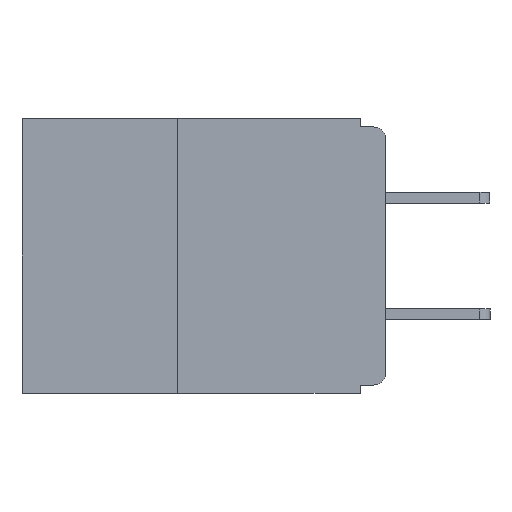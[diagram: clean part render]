
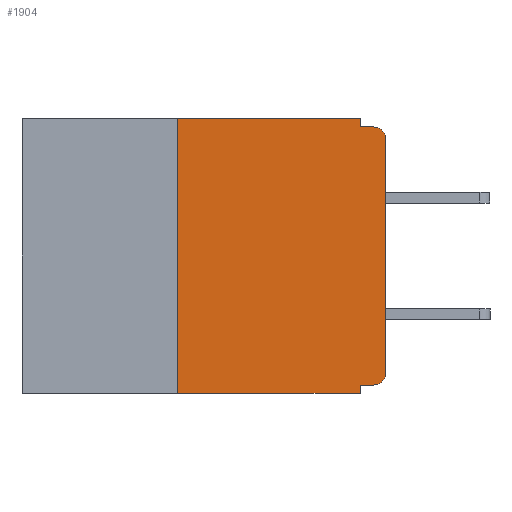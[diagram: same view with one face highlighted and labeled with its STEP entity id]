
A CAD part, left-side view. The second image highlights one B-rep face of the part: STEP entity #1904.
In plain terms, the highlighted planar face has unit normal (-1, 0, 0).
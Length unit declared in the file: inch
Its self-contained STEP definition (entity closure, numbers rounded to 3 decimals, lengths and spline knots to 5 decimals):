
#303 = LINE ( 'NONE', #9663, #15278 ) ;
#371 = DIRECTION ( 'NONE',  ( 0., -1., 0. ) ) ;
#398 = CARTESIAN_POINT ( 'NONE',  ( 0., 0.031, 0. ) ) ;
#621 = DIRECTION ( 'NONE',  ( 0., -1., 0. ) ) ;
#967 = CARTESIAN_POINT ( 'NONE',  ( 0., 0.031, 0. ) ) ;
#1322 = CARTESIAN_POINT ( 'NONE',  ( 0., 0.015, -0.01 ) ) ;
#1361 = ORIENTED_EDGE ( 'NONE', *, *, #13962, .F. ) ;
#1904 = ADVANCED_FACE ( 'NONE', ( #8468 ), #15203, .F. ) ;
#2011 = CARTESIAN_POINT ( 'NONE',  ( 0., 0., -0.01 ) ) ;
#2125 = EDGE_LOOP ( 'NONE', ( #11844, #4583, #15619, #1361, #17449, #3316, #15454, #16889, #7961, #3731 ) ) ;
#2155 = DIRECTION ( 'NONE',  ( 0., 0., -1. ) ) ;
#3179 = CARTESIAN_POINT ( 'NONE',  ( 0., 0., -0.32 ) ) ;
#3259 = EDGE_CURVE ( 'NONE', #14240, #4180, #303, .T. ) ;
#3316 = ORIENTED_EDGE ( 'NONE', *, *, #17356, .F. ) ;
#3629 = VECTOR ( 'NONE', #3844, 39.37008 ) ;
#3650 = VECTOR ( 'NONE', #8616, 39.37008 ) ;
#3731 = ORIENTED_EDGE ( 'NONE', *, *, #3774, .T. ) ;
#3774 = EDGE_CURVE ( 'NONE', #13716, #15517, #13605, .T. ) ;
#3844 = DIRECTION ( 'NONE',  ( 0., 0., 1. ) ) ;
#3889 = DIRECTION ( 'NONE',  ( -1., 0., 0. ) ) ;
#4069 = LINE ( 'NONE', #3179, #3650 ) ;
#4118 = CARTESIAN_POINT ( 'NONE',  ( 0., 0.031, -0.33 ) ) ;
#4129 = VERTEX_POINT ( 'NONE', #1322 ) ;
#4180 = VERTEX_POINT ( 'NONE', #398 ) ;
#4583 = ORIENTED_EDGE ( 'NONE', *, *, #14021, .T. ) ;
#5123 = CARTESIAN_POINT ( 'NONE',  ( 0., 0.25, -0.33 ) ) ;
#5500 = VECTOR ( 'NONE', #10630, 39.37008 ) ;
#6365 = VERTEX_POINT ( 'NONE', #8683 ) ;
#6966 = EDGE_CURVE ( 'NONE', #11649, #13072, #15806, .T. ) ;
#7050 = CARTESIAN_POINT ( 'NONE',  ( 0., 0., -0.025 ) ) ;
#7576 = CARTESIAN_POINT ( 'NONE',  ( 0., 0.031, -0.33 ) ) ;
#7876 = EDGE_CURVE ( 'NONE', #15517, #9185, #15364, .T. ) ;
#7961 = ORIENTED_EDGE ( 'NONE', *, *, #8109, .F. ) ;
#8109 = EDGE_CURVE ( 'NONE', #13716, #6365, #4069, .T. ) ;
#8189 = DIRECTION ( 'NONE',  ( 0., 0., -1. ) ) ;
#8252 = DIRECTION ( 'NONE',  ( -1., 0., 0. ) ) ;
#8309 = CARTESIAN_POINT ( 'NONE',  ( 0., 0.015, -0.305 ) ) ;
#8390 = AXIS2_PLACEMENT_3D ( 'NONE', #8309, #8252, #8189 ) ;
#8468 = FACE_OUTER_BOUND ( 'NONE', #2125, .T. ) ;
#8577 = CARTESIAN_POINT ( 'NONE',  ( 0., 0.015, -0.32 ) ) ;
#8616 = DIRECTION ( 'NONE',  ( 0., 1., 0. ) ) ;
#8683 = CARTESIAN_POINT ( 'NONE',  ( 0., 0.031, -0.32 ) ) ;
#8833 = EDGE_CURVE ( 'NONE', #12652, #4129, #13897, .T. ) ;
#9113 = LINE ( 'NONE', #15966, #5500 ) ;
#9120 = DIRECTION ( 'NONE',  ( 0., 0., -1. ) ) ;
#9185 = VERTEX_POINT ( 'NONE', #7050 ) ;
#9663 = CARTESIAN_POINT ( 'NONE',  ( 0., 0.437, 0. ) ) ;
#9790 = CIRCLE ( 'NONE', #15237, 0.015 ) ;
#10630 = DIRECTION ( 'NONE',  ( 0., 0., 1. ) ) ;
#10696 = CARTESIAN_POINT ( 'NONE',  ( 0., 0., 0. ) ) ;
#10961 = DIRECTION ( 'NONE',  ( 0., -1., 0. ) ) ;
#11154 = CARTESIAN_POINT ( 'NONE',  ( 0., 0.25, 0. ) ) ;
#11378 = CARTESIAN_POINT ( 'NONE',  ( 0., 0.437, -0.33 ) ) ;
#11521 = EDGE_CURVE ( 'NONE', #6365, #13072, #13344, .T. ) ;
#11560 = CARTESIAN_POINT ( 'NONE',  ( 0., 0.031, -0.01 ) ) ;
#11649 = VERTEX_POINT ( 'NONE', #5123 ) ;
#11844 = ORIENTED_EDGE ( 'NONE', *, *, #7876, .T. ) ;
#12132 = CARTESIAN_POINT ( 'NONE',  ( 0., 0.015, -0.025 ) ) ;
#12652 = VERTEX_POINT ( 'NONE', #11560 ) ;
#12926 = VECTOR ( 'NONE', #2155, 39.37008 ) ;
#13072 = VERTEX_POINT ( 'NONE', #4118 ) ;
#13344 = LINE ( 'NONE', #7576, #12926 ) ;
#13488 = DIRECTION ( 'NONE',  ( 0., 0., -1. ) ) ;
#13605 = CIRCLE ( 'NONE', #8390, 0.015 ) ;
#13716 = VERTEX_POINT ( 'NONE', #8577 ) ;
#13867 = VECTOR ( 'NONE', #9120, 39.37008 ) ;
#13897 = LINE ( 'NONE', #2011, #16980 ) ;
#13962 = EDGE_CURVE ( 'NONE', #4180, #12652, #17333, .T. ) ;
#14021 = EDGE_CURVE ( 'NONE', #9185, #4129, #9790, .T. ) ;
#14240 = VERTEX_POINT ( 'NONE', #11154 ) ;
#15203 = PLANE ( 'NONE',  #15377 ) ;
#15221 = DIRECTION ( 'NONE',  ( 0., 0., -1. ) ) ;
#15237 = AXIS2_PLACEMENT_3D ( 'NONE', #12132, #3889, #13488 ) ;
#15278 = VECTOR ( 'NONE', #10961, 39.37008 ) ;
#15280 = DIRECTION ( 'NONE',  ( 1., 0., 0. ) ) ;
#15343 = CARTESIAN_POINT ( 'NONE',  ( 0., 0.437, 0. ) ) ;
#15364 = LINE ( 'NONE', #10696, #3629 ) ;
#15377 = AXIS2_PLACEMENT_3D ( 'NONE', #15343, #15280, #15221 ) ;
#15397 = VECTOR ( 'NONE', #371, 39.37008 ) ;
#15454 = ORIENTED_EDGE ( 'NONE', *, *, #6966, .T. ) ;
#15460 = CARTESIAN_POINT ( 'NONE',  ( 0., 0., -0.305 ) ) ;
#15517 = VERTEX_POINT ( 'NONE', #15460 ) ;
#15619 = ORIENTED_EDGE ( 'NONE', *, *, #8833, .F. ) ;
#15806 = LINE ( 'NONE', #11378, #15397 ) ;
#15966 = CARTESIAN_POINT ( 'NONE',  ( 0., 0.25, -0.33 ) ) ;
#16889 = ORIENTED_EDGE ( 'NONE', *, *, #11521, .F. ) ;
#16980 = VECTOR ( 'NONE', #621, 39.37008 ) ;
#17333 = LINE ( 'NONE', #967, #13867 ) ;
#17356 = EDGE_CURVE ( 'NONE', #11649, #14240, #9113, .T. ) ;
#17449 = ORIENTED_EDGE ( 'NONE', *, *, #3259, .F. ) ;
